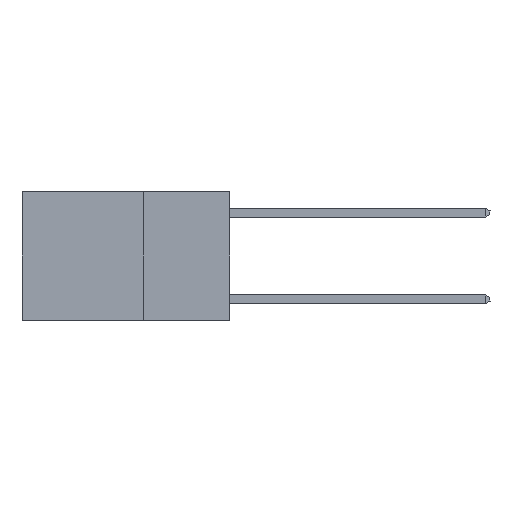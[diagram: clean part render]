
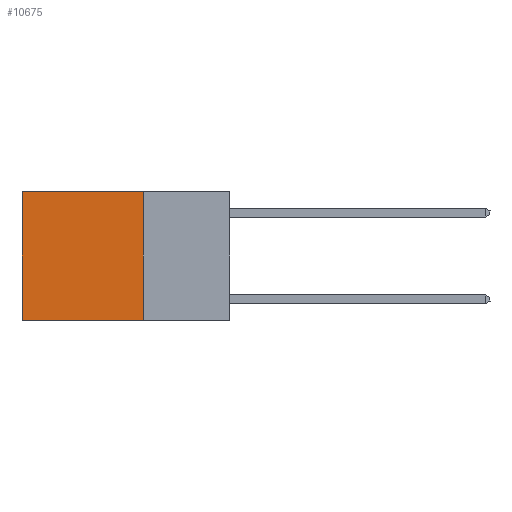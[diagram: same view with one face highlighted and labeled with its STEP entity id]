
A CAD part, left-side view. The second image highlights one B-rep face of the part: STEP entity #10675.
In plain terms, the highlighted planar face has unit normal (-1, 0, 0).
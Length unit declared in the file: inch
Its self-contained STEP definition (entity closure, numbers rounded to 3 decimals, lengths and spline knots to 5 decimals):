
#865 = EDGE_CURVE ( 'NONE', #24944, #11678, #1317, .T. ) ;
#930 = DIRECTION ( 'NONE',  ( 0., 0., -1. ) ) ;
#1317 = LINE ( 'NONE', #10009, #4566 ) ;
#1723 = EDGE_CURVE ( 'NONE', #24944, #26481, #24689, .T. ) ;
#3488 = EDGE_CURVE ( 'NONE', #11678, #22684, #25412, .T. ) ;
#3506 = DIRECTION ( 'NONE',  ( 0., 1., 0. ) ) ;
#4566 = VECTOR ( 'NONE', #3506, 39.37008 ) ;
#4633 = CARTESIAN_POINT ( 'NONE',  ( 0.2625, 0.25, 0. ) ) ;
#7981 = CARTESIAN_POINT ( 'NONE',  ( 0.2625, 0.6, 0. ) ) ;
#8235 = CARTESIAN_POINT ( 'NONE',  ( 0.2625, 0.25, -0.37 ) ) ;
#8643 = FACE_OUTER_BOUND ( 'NONE', #25149, .T. ) ;
#9365 = ORIENTED_EDGE ( 'NONE', *, *, #1723, .F. ) ;
#10009 = CARTESIAN_POINT ( 'NONE',  ( 0.2625, 0.25, 0. ) ) ;
#10285 = CARTESIAN_POINT ( 'NONE',  ( 0.2625, 0.25, -0.37 ) ) ;
#10644 = EDGE_CURVE ( 'NONE', #26481, #22684, #19043, .T. ) ;
#10675 = ADVANCED_FACE ( 'NONE', ( #8643 ), #19900, .F. ) ;
#11123 = DIRECTION ( 'NONE',  ( 0., 1., 0. ) ) ;
#11164 = ORIENTED_EDGE ( 'NONE', *, *, #3488, .T. ) ;
#11678 = VERTEX_POINT ( 'NONE', #22858 ) ;
#19043 = LINE ( 'NONE', #10285, #20246 ) ;
#19504 = VECTOR ( 'NONE', #930, 39.37008 ) ;
#19900 = PLANE ( 'NONE',  #24885 ) ;
#20246 = VECTOR ( 'NONE', #11123, 39.37008 ) ;
#20973 = CARTESIAN_POINT ( 'NONE',  ( 0.2625, 0.25, 0. ) ) ;
#21580 = VECTOR ( 'NONE', #22515, 39.37008 ) ;
#21950 = ORIENTED_EDGE ( 'NONE', *, *, #10644, .F. ) ;
#22515 = DIRECTION ( 'NONE',  ( 0., 0., -1. ) ) ;
#22684 = VERTEX_POINT ( 'NONE', #22954 ) ;
#22858 = CARTESIAN_POINT ( 'NONE',  ( 0.2625, 0.6, 0. ) ) ;
#22954 = CARTESIAN_POINT ( 'NONE',  ( 0.2625, 0.6, -0.37 ) ) ;
#23945 = ORIENTED_EDGE ( 'NONE', *, *, #865, .T. ) ;
#24278 = DIRECTION ( 'NONE',  ( 1., 0., 0. ) ) ;
#24430 = DIRECTION ( 'NONE',  ( 0., 0., -1. ) ) ;
#24689 = LINE ( 'NONE', #4633, #21580 ) ;
#24885 = AXIS2_PLACEMENT_3D ( 'NONE', #26626, #24278, #24430 ) ;
#24944 = VERTEX_POINT ( 'NONE', #20973 ) ;
#25149 = EDGE_LOOP ( 'NONE', ( #11164, #21950, #9365, #23945 ) ) ;
#25412 = LINE ( 'NONE', #7981, #19504 ) ;
#26481 = VERTEX_POINT ( 'NONE', #8235 ) ;
#26626 = CARTESIAN_POINT ( 'NONE',  ( 0.2625, 0.25, 0. ) ) ;
